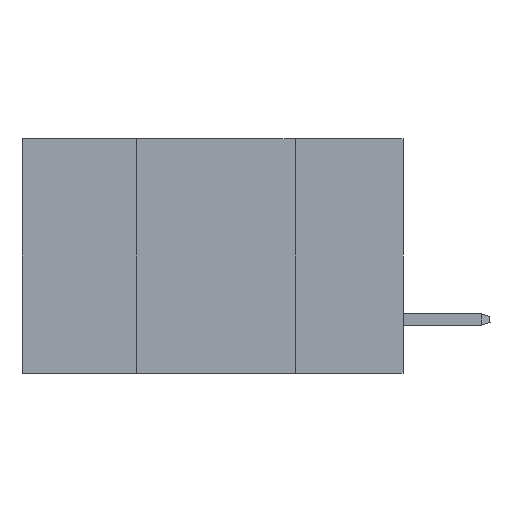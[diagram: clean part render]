
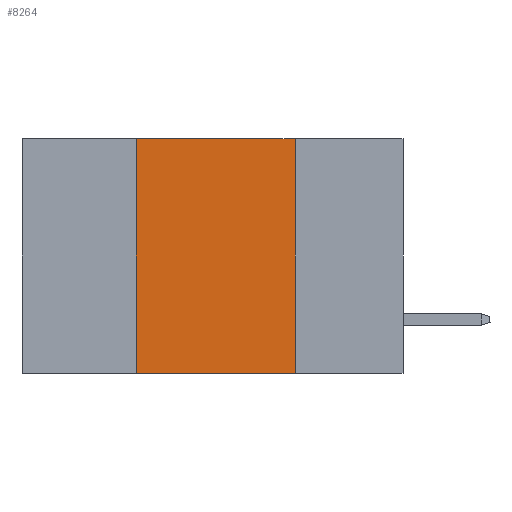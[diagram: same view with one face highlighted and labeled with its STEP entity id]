
A CAD part, left-side view. The second image highlights one B-rep face of the part: STEP entity #8264.
In plain terms, the highlighted planar face has unit normal (-1, 0, 0).
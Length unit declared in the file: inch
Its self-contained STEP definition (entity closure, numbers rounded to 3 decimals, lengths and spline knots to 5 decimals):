
#696 = DIRECTION ( 'NONE',  ( 0., 0., -1. ) ) ;
#1227 = CARTESIAN_POINT ( 'NONE',  ( 0., 0.6, -0.37 ) ) ;
#2280 = EDGE_LOOP ( 'NONE', ( #9894, #13524, #3953, #22518 ) ) ;
#2738 = DIRECTION ( 'NONE',  ( 0., 0., -1. ) ) ;
#3953 = ORIENTED_EDGE ( 'NONE', *, *, #15278, .F. ) ;
#4283 = PLANE ( 'NONE',  #6624 ) ;
#4475 = LINE ( 'NONE', #6691, #9018 ) ;
#5682 = VECTOR ( 'NONE', #22689, 39.37008 ) ;
#6624 = AXIS2_PLACEMENT_3D ( 'NONE', #11550, #13887, #696 ) ;
#6691 = CARTESIAN_POINT ( 'NONE',  ( 0., 0.17, 0. ) ) ;
#7012 = DIRECTION ( 'NONE',  ( 0., -1., 0. ) ) ;
#7793 = VERTEX_POINT ( 'NONE', #15074 ) ;
#7872 = VECTOR ( 'NONE', #17832, 39.37008 ) ;
#7947 = VERTEX_POINT ( 'NONE', #13922 ) ;
#8264 = ADVANCED_FACE ( 'NONE', ( #21302 ), #4283, .F. ) ;
#8442 = CARTESIAN_POINT ( 'NONE',  ( 0., 0.6, 0. ) ) ;
#8541 = VECTOR ( 'NONE', #7012, 39.37008 ) ;
#9018 = VECTOR ( 'NONE', #2738, 39.37008 ) ;
#9894 = ORIENTED_EDGE ( 'NONE', *, *, #22197, .F. ) ;
#10184 = VERTEX_POINT ( 'NONE', #18204 ) ;
#10913 = CARTESIAN_POINT ( 'NONE',  ( 0., 0.17, 0. ) ) ;
#11473 = CARTESIAN_POINT ( 'NONE',  ( 0., 0.42, 0. ) ) ;
#11550 = CARTESIAN_POINT ( 'NONE',  ( 0., 0.6, 0. ) ) ;
#12442 = LINE ( 'NONE', #1227, #8541 ) ;
#13524 = ORIENTED_EDGE ( 'NONE', *, *, #23519, .F. ) ;
#13887 = DIRECTION ( 'NONE',  ( 1., 0., 0. ) ) ;
#13922 = CARTESIAN_POINT ( 'NONE',  ( 0., 0.42, -0.37 ) ) ;
#14360 = VERTEX_POINT ( 'NONE', #10913 ) ;
#15074 = CARTESIAN_POINT ( 'NONE',  ( 0., 0.42, 0. ) ) ;
#15278 = EDGE_CURVE ( 'NONE', #7947, #7793, #17612, .T. ) ;
#17612 = LINE ( 'NONE', #11473, #5682 ) ;
#17832 = DIRECTION ( 'NONE',  ( 0., -1., 0. ) ) ;
#18204 = CARTESIAN_POINT ( 'NONE',  ( 0., 0.17, -0.37 ) ) ;
#18921 = EDGE_CURVE ( 'NONE', #7947, #10184, #12442, .T. ) ;
#20055 = LINE ( 'NONE', #8442, #7872 ) ;
#21302 = FACE_OUTER_BOUND ( 'NONE', #2280, .T. ) ;
#22197 = EDGE_CURVE ( 'NONE', #14360, #10184, #4475, .T. ) ;
#22518 = ORIENTED_EDGE ( 'NONE', *, *, #18921, .T. ) ;
#22689 = DIRECTION ( 'NONE',  ( 0., 0., 1. ) ) ;
#23519 = EDGE_CURVE ( 'NONE', #7793, #14360, #20055, .T. ) ;
